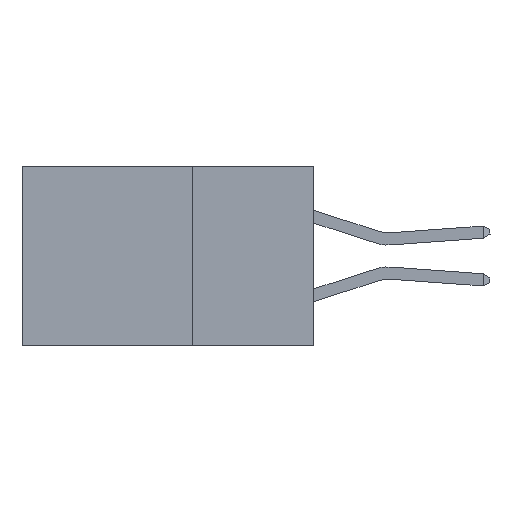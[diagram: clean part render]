
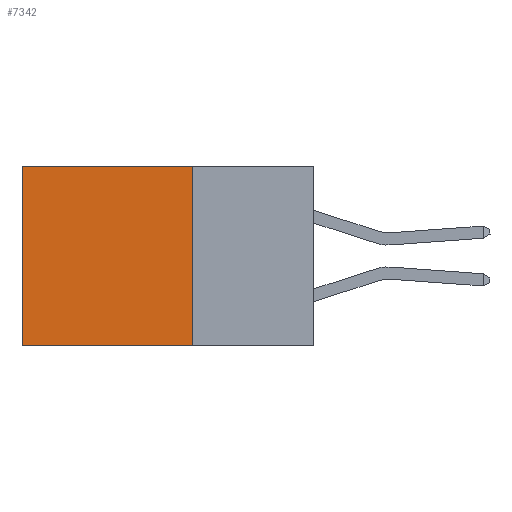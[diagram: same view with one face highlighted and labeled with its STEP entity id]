
A CAD part, left-side view. The second image highlights one B-rep face of the part: STEP entity #7342.
In plain terms, the highlighted planar face has unit normal (-1, 0, 0).
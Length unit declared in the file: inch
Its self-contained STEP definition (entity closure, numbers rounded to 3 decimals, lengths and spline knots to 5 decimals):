
#158 = VECTOR ( 'NONE', #9178, 39.37008 ) ;
#248 = VERTEX_POINT ( 'NONE', #5409 ) ;
#257 = EDGE_CURVE ( 'NONE', #9351, #6270, #4371, .T. ) ;
#396 = LINE ( 'NONE', #10035, #158 ) ;
#702 = LINE ( 'NONE', #6048, #7549 ) ;
#827 = EDGE_LOOP ( 'NONE', ( #2009, #7162, #4643, #8921 ) ) ;
#924 = PLANE ( 'NONE',  #3044 ) ;
#949 = DIRECTION ( 'NONE',  ( 0., 0., -1. ) ) ;
#984 = EDGE_CURVE ( 'NONE', #6270, #3411, #702, .T. ) ;
#1304 = DIRECTION ( 'NONE',  ( 0., 0., -1. ) ) ;
#1611 = VECTOR ( 'NONE', #5511, 39.37008 ) ;
#2009 = ORIENTED_EDGE ( 'NONE', *, *, #984, .T. ) ;
#3044 = AXIS2_PLACEMENT_3D ( 'NONE', #8080, #5719, #949 ) ;
#3411 = VERTEX_POINT ( 'NONE', #3817 ) ;
#3442 = FACE_OUTER_BOUND ( 'NONE', #827, .T. ) ;
#3817 = CARTESIAN_POINT ( 'NONE',  ( 0.2875, 0.6, -0.37 ) ) ;
#3957 = DIRECTION ( 'NONE',  ( 0., 1., 0. ) ) ;
#3967 = CARTESIAN_POINT ( 'NONE',  ( 0.2875, 0.25, 0. ) ) ;
#4316 = EDGE_CURVE ( 'NONE', #9351, #248, #396, .T. ) ;
#4371 = LINE ( 'NONE', #4607, #5342 ) ;
#4607 = CARTESIAN_POINT ( 'NONE',  ( 0.2875, 0.25, 0. ) ) ;
#4643 = ORIENTED_EDGE ( 'NONE', *, *, #4316, .F. ) ;
#5342 = VECTOR ( 'NONE', #3957, 39.37008 ) ;
#5409 = CARTESIAN_POINT ( 'NONE',  ( 0.2875, 0.25, -0.37 ) ) ;
#5511 = DIRECTION ( 'NONE',  ( 0., 1., 0. ) ) ;
#5719 = DIRECTION ( 'NONE',  ( 1., 0., 0. ) ) ;
#6048 = CARTESIAN_POINT ( 'NONE',  ( 0.2875, 0.6, 0. ) ) ;
#6270 = VERTEX_POINT ( 'NONE', #10309 ) ;
#7162 = ORIENTED_EDGE ( 'NONE', *, *, #8218, .F. ) ;
#7342 = ADVANCED_FACE ( 'NONE', ( #3442 ), #924, .F. ) ;
#7549 = VECTOR ( 'NONE', #1304, 39.37008 ) ;
#8080 = CARTESIAN_POINT ( 'NONE',  ( 0.2875, 0.25, 0. ) ) ;
#8218 = EDGE_CURVE ( 'NONE', #248, #3411, #8955, .T. ) ;
#8664 = CARTESIAN_POINT ( 'NONE',  ( 0.2875, 0.25, -0.37 ) ) ;
#8921 = ORIENTED_EDGE ( 'NONE', *, *, #257, .T. ) ;
#8955 = LINE ( 'NONE', #8664, #1611 ) ;
#9178 = DIRECTION ( 'NONE',  ( 0., 0., -1. ) ) ;
#9351 = VERTEX_POINT ( 'NONE', #3967 ) ;
#10035 = CARTESIAN_POINT ( 'NONE',  ( 0.2875, 0.25, 0. ) ) ;
#10309 = CARTESIAN_POINT ( 'NONE',  ( 0.2875, 0.6, 0. ) ) ;
